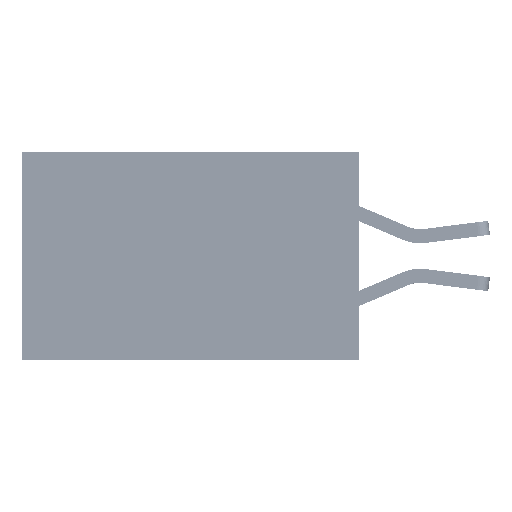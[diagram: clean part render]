
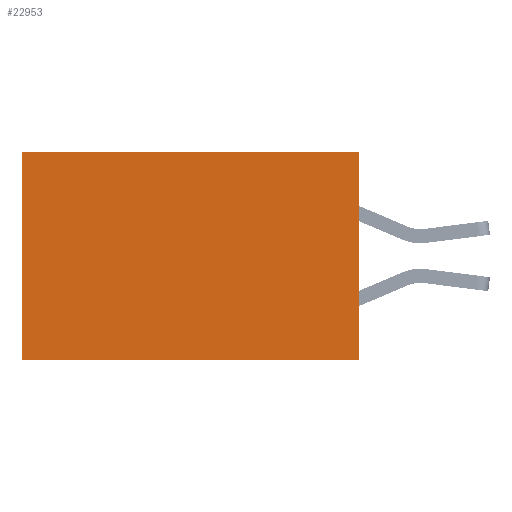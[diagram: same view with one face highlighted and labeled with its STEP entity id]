
A CAD part, left-side view. The second image highlights one B-rep face of the part: STEP entity #22953.
In plain terms, the highlighted planar face has unit normal (-1, 0, 0).
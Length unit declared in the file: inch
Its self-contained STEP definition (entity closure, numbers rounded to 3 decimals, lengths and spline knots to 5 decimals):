
#1872 = LINE ( 'NONE', #22990, #26745 ) ;
#2675 = VECTOR ( 'NONE', #9038, 39.37008 ) ;
#4210 = AXIS2_PLACEMENT_3D ( 'NONE', #9759, #13075, #36250 ) ;
#4610 = EDGE_CURVE ( 'NONE', #14551, #30029, #1872, .T. ) ;
#5705 = EDGE_CURVE ( 'NONE', #27274, #14551, #37551, .T. ) ;
#7347 = EDGE_CURVE ( 'NONE', #14418, #30029, #22903, .T. ) ;
#9034 = DIRECTION ( 'NONE',  ( 0., 0., -1. ) ) ;
#9038 = DIRECTION ( 'NONE',  ( 0., 1., 0. ) ) ;
#9759 = CARTESIAN_POINT ( 'NONE',  ( 0.2875, 0., 0. ) ) ;
#12506 = ORIENTED_EDGE ( 'NONE', *, *, #5705, .F. ) ;
#13075 = DIRECTION ( 'NONE',  ( 1., 0., 0. ) ) ;
#13551 = VECTOR ( 'NONE', #9034, 39.37008 ) ;
#14418 = VERTEX_POINT ( 'NONE', #25445 ) ;
#14551 = VERTEX_POINT ( 'NONE', #19217 ) ;
#15546 = CARTESIAN_POINT ( 'NONE',  ( 0.2875, 0.6, 0. ) ) ;
#18323 = CARTESIAN_POINT ( 'NONE',  ( 0.2875, 0., 0. ) ) ;
#19217 = CARTESIAN_POINT ( 'NONE',  ( 0.2875, 0., -0.37 ) ) ;
#19274 = DIRECTION ( 'NONE',  ( 0., 0., -1. ) ) ;
#19577 = EDGE_CURVE ( 'NONE', #27274, #14418, #36820, .T. ) ;
#22903 = LINE ( 'NONE', #15546, #13551 ) ;
#22953 = ADVANCED_FACE ( 'NONE', ( #23948 ), #32641, .F. ) ;
#22990 = CARTESIAN_POINT ( 'NONE',  ( 0.2875, 0., -0.37 ) ) ;
#23442 = ORIENTED_EDGE ( 'NONE', *, *, #19577, .T. ) ;
#23948 = FACE_OUTER_BOUND ( 'NONE', #33663, .T. ) ;
#25445 = CARTESIAN_POINT ( 'NONE',  ( 0.2875, 0.6, 0. ) ) ;
#26485 = DIRECTION ( 'NONE',  ( 0., 1., 0. ) ) ;
#26745 = VECTOR ( 'NONE', #26485, 39.37008 ) ;
#27245 = ORIENTED_EDGE ( 'NONE', *, *, #7347, .T. ) ;
#27274 = VERTEX_POINT ( 'NONE', #30296 ) ;
#28769 = VECTOR ( 'NONE', #19274, 39.37008 ) ;
#30029 = VERTEX_POINT ( 'NONE', #34075 ) ;
#30296 = CARTESIAN_POINT ( 'NONE',  ( 0.2875, 0., 0. ) ) ;
#32257 = ORIENTED_EDGE ( 'NONE', *, *, #4610, .F. ) ;
#32582 = CARTESIAN_POINT ( 'NONE',  ( 0.2875, 0., 0. ) ) ;
#32641 = PLANE ( 'NONE',  #4210 ) ;
#33663 = EDGE_LOOP ( 'NONE', ( #27245, #32257, #12506, #23442 ) ) ;
#34075 = CARTESIAN_POINT ( 'NONE',  ( 0.2875, 0.6, -0.37 ) ) ;
#36250 = DIRECTION ( 'NONE',  ( 0., 0., -1. ) ) ;
#36820 = LINE ( 'NONE', #18323, #2675 ) ;
#37551 = LINE ( 'NONE', #32582, #28769 ) ;
